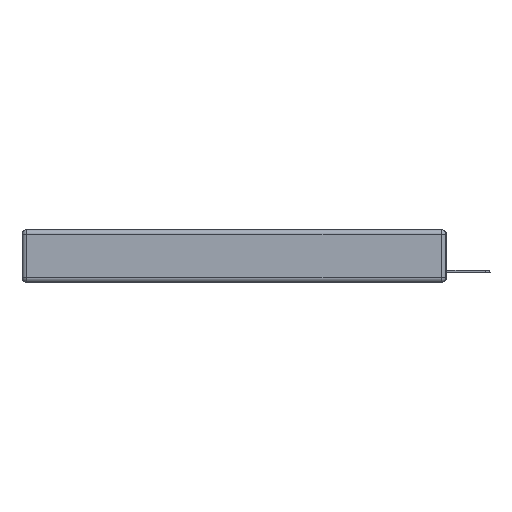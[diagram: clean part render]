
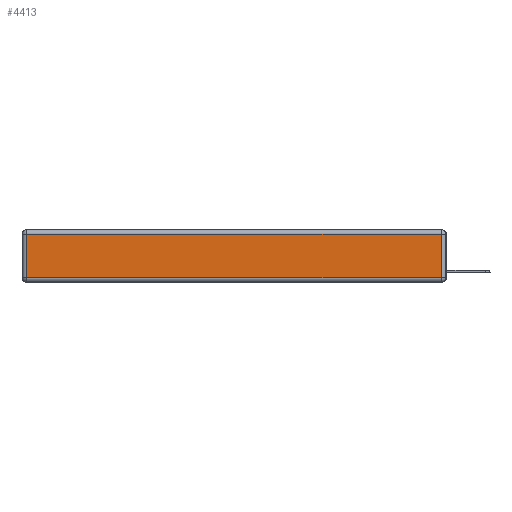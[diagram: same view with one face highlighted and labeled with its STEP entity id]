
A CAD part, left-side view. The second image highlights one B-rep face of the part: STEP entity #4413.
In plain terms, the highlighted planar face has unit normal (-1, 0, 0).
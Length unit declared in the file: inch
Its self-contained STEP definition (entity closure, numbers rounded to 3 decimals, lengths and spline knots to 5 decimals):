
#61 = VECTOR ( 'NONE', #17129, 39.37008 ) ;
#68 = FACE_OUTER_BOUND ( 'NONE', #5969, .T. ) ;
#810 = CARTESIAN_POINT ( 'NONE',  ( 0., 2.72, -0.343 ) ) ;
#1466 = DIRECTION ( 'NONE',  ( -1., 0., 0. ) ) ;
#2024 = VERTEX_POINT ( 'NONE', #8275 ) ;
#2311 = EDGE_CURVE ( 'NONE', #2024, #9984, #7851, .T. ) ;
#2428 = CARTESIAN_POINT ( 'NONE',  ( 0., 0.03, -0.03 ) ) ;
#2770 = VECTOR ( 'NONE', #7496, 39.37008 ) ;
#4413 = ADVANCED_FACE ( 'NONE', ( #68 ), #12786, .T. ) ;
#5969 = EDGE_LOOP ( 'NONE', ( #20849, #18295, #11522, #10552 ) ) ;
#6649 = LINE ( 'NONE', #7226, #61 ) ;
#6661 = CARTESIAN_POINT ( 'NONE',  ( 0., 2.75, -0.03 ) ) ;
#7226 = CARTESIAN_POINT ( 'NONE',  ( 0., 0.03, -0.343 ) ) ;
#7475 = CARTESIAN_POINT ( 'NONE',  ( 0., 0.03, -0.313 ) ) ;
#7496 = DIRECTION ( 'NONE',  ( 0., 0., -1. ) ) ;
#7851 = LINE ( 'NONE', #810, #2770 ) ;
#8226 = DIRECTION ( 'NONE',  ( 0., 0., 1. ) ) ;
#8275 = CARTESIAN_POINT ( 'NONE',  ( 0., 2.72, -0.03 ) ) ;
#8810 = CARTESIAN_POINT ( 'NONE',  ( 0., 2.72, -0.313 ) ) ;
#9948 = DIRECTION ( 'NONE',  ( 0., 1., 0. ) ) ;
#9984 = VERTEX_POINT ( 'NONE', #8810 ) ;
#10552 = ORIENTED_EDGE ( 'NONE', *, *, #2311, .T. ) ;
#10846 = EDGE_CURVE ( 'NONE', #9984, #20350, #12832, .T. ) ;
#11102 = EDGE_CURVE ( 'NONE', #11384, #2024, #12562, .T. ) ;
#11384 = VERTEX_POINT ( 'NONE', #2428 ) ;
#11522 = ORIENTED_EDGE ( 'NONE', *, *, #11102, .T. ) ;
#12310 = VECTOR ( 'NONE', #15592, 39.37008 ) ;
#12323 = EDGE_CURVE ( 'NONE', #20350, #11384, #6649, .T. ) ;
#12562 = LINE ( 'NONE', #6661, #15636 ) ;
#12786 = PLANE ( 'NONE',  #20661 ) ;
#12832 = LINE ( 'NONE', #19125, #12310 ) ;
#15592 = DIRECTION ( 'NONE',  ( 0., -1., 0. ) ) ;
#15636 = VECTOR ( 'NONE', #9948, 39.37008 ) ;
#17129 = DIRECTION ( 'NONE',  ( 0., 0., 1. ) ) ;
#18295 = ORIENTED_EDGE ( 'NONE', *, *, #12323, .T. ) ;
#19125 = CARTESIAN_POINT ( 'NONE',  ( 0., 0., -0.313 ) ) ;
#20350 = VERTEX_POINT ( 'NONE', #7475 ) ;
#20661 = AXIS2_PLACEMENT_3D ( 'NONE', #21006, #1466, #8226 ) ;
#20849 = ORIENTED_EDGE ( 'NONE', *, *, #10846, .T. ) ;
#21006 = CARTESIAN_POINT ( 'NONE',  ( 0., 0., -0.343 ) ) ;
